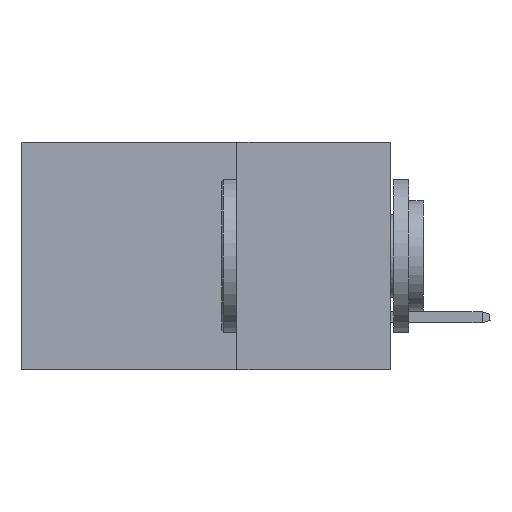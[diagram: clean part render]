
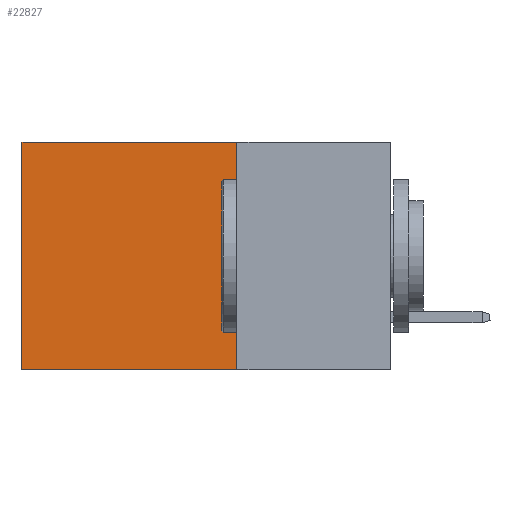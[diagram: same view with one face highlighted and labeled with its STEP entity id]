
A CAD part, left-side view. The second image highlights one B-rep face of the part: STEP entity #22827.
In plain terms, the highlighted planar face has unit normal (-1, 0, 0).
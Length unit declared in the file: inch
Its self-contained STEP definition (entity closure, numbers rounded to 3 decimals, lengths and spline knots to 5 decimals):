
#380 = VECTOR ( 'NONE', #16876, 39.37008 ) ;
#807 = CARTESIAN_POINT ( 'NONE',  ( 0.2875, 0.25, 0. ) ) ;
#2064 = EDGE_CURVE ( 'NONE', #7557, #5585, #15073, .T. ) ;
#2080 = DIRECTION ( 'NONE',  ( 0., 0., -1. ) ) ;
#2122 = ORIENTED_EDGE ( 'NONE', *, *, #11042, .F. ) ;
#2780 = ORIENTED_EDGE ( 'NONE', *, *, #2064, .T. ) ;
#3213 = LINE ( 'NONE', #18441, #22055 ) ;
#3429 = CARTESIAN_POINT ( 'NONE',  ( 0.2875, 0.25, 0. ) ) ;
#4381 = EDGE_LOOP ( 'NONE', ( #4428, #2122, #13591, #2780 ) ) ;
#4428 = ORIENTED_EDGE ( 'NONE', *, *, #18006, .T. ) ;
#4458 = FACE_OUTER_BOUND ( 'NONE', #4381, .T. ) ;
#5552 = CARTESIAN_POINT ( 'NONE',  ( 0.2875, 0.25, -0.37 ) ) ;
#5585 = VERTEX_POINT ( 'NONE', #19258 ) ;
#6201 = VECTOR ( 'NONE', #18095, 39.37008 ) ;
#6786 = LINE ( 'NONE', #3429, #6201 ) ;
#7557 = VERTEX_POINT ( 'NONE', #807 ) ;
#7862 = EDGE_CURVE ( 'NONE', #7557, #23476, #6786, .T. ) ;
#8476 = DIRECTION ( 'NONE',  ( 1., 0., 0. ) ) ;
#8776 = VECTOR ( 'NONE', #19829, 39.37008 ) ;
#9346 = CARTESIAN_POINT ( 'NONE',  ( 0.2875, 0.6, -0.37 ) ) ;
#9793 = LINE ( 'NONE', #5552, #380 ) ;
#10970 = CARTESIAN_POINT ( 'NONE',  ( 0.2875, 0.25, 0. ) ) ;
#11042 = EDGE_CURVE ( 'NONE', #23476, #13547, #9793, .T. ) ;
#12067 = PLANE ( 'NONE',  #23650 ) ;
#12151 = CARTESIAN_POINT ( 'NONE',  ( 0.2875, 0.25, 0. ) ) ;
#13547 = VERTEX_POINT ( 'NONE', #9346 ) ;
#13591 = ORIENTED_EDGE ( 'NONE', *, *, #7862, .F. ) ;
#15073 = LINE ( 'NONE', #10970, #8776 ) ;
#16876 = DIRECTION ( 'NONE',  ( 0., 1., 0. ) ) ;
#18006 = EDGE_CURVE ( 'NONE', #5585, #13547, #3213, .T. ) ;
#18095 = DIRECTION ( 'NONE',  ( 0., 0., -1. ) ) ;
#18441 = CARTESIAN_POINT ( 'NONE',  ( 0.2875, 0.6, 0. ) ) ;
#19258 = CARTESIAN_POINT ( 'NONE',  ( 0.2875, 0.6, 0. ) ) ;
#19829 = DIRECTION ( 'NONE',  ( 0., 1., 0. ) ) ;
#21260 = DIRECTION ( 'NONE',  ( 0., 0., -1. ) ) ;
#21657 = CARTESIAN_POINT ( 'NONE',  ( 0.2875, 0.25, -0.37 ) ) ;
#22055 = VECTOR ( 'NONE', #2080, 39.37008 ) ;
#22827 = ADVANCED_FACE ( 'NONE', ( #4458 ), #12067, .F. ) ;
#23476 = VERTEX_POINT ( 'NONE', #21657 ) ;
#23650 = AXIS2_PLACEMENT_3D ( 'NONE', #12151, #8476, #21260 ) ;
